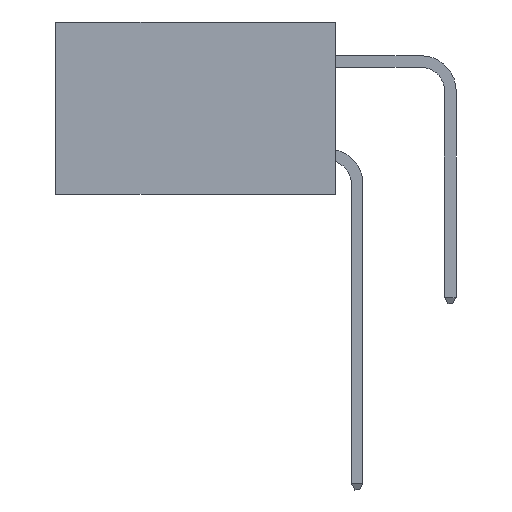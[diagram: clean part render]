
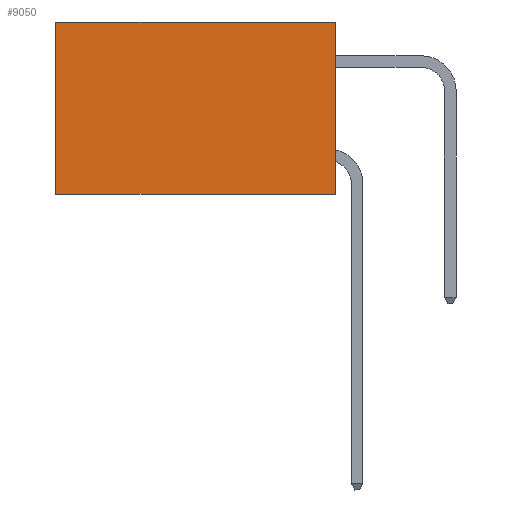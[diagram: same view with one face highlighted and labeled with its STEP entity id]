
A CAD part, left-side view. The second image highlights one B-rep face of the part: STEP entity #9050.
In plain terms, the highlighted planar face has unit normal (-1, 0, 0).
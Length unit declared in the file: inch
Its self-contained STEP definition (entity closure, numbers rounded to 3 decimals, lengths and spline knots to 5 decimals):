
#246 = DIRECTION ( 'NONE',  ( 1., 0., 0. ) ) ;
#2135 = CARTESIAN_POINT ( 'NONE',  ( 0.2875, 0.6, -0.37 ) ) ;
#3579 = VERTEX_POINT ( 'NONE', #6731 ) ;
#5837 = ORIENTED_EDGE ( 'NONE', *, *, #15060, .T. ) ;
#6731 = CARTESIAN_POINT ( 'NONE',  ( 0.2875, 0., -0.37 ) ) ;
#9050 = ADVANCED_FACE ( 'NONE', ( #21233 ), #11220, .F. ) ;
#9184 = DIRECTION ( 'NONE',  ( 0., 1., 0. ) ) ;
#10200 = CARTESIAN_POINT ( 'NONE',  ( 0.2875, 0., 0. ) ) ;
#10990 = DIRECTION ( 'NONE',  ( 0., 0., -1. ) ) ;
#11158 = DIRECTION ( 'NONE',  ( 0., 0., -1. ) ) ;
#11220 = PLANE ( 'NONE',  #15817 ) ;
#11333 = EDGE_CURVE ( 'NONE', #24802, #27019, #31255, .T. ) ;
#13932 = CARTESIAN_POINT ( 'NONE',  ( 0.2875, 0., 0. ) ) ;
#15060 = EDGE_CURVE ( 'NONE', #20950, #24802, #25091, .T. ) ;
#15817 = AXIS2_PLACEMENT_3D ( 'NONE', #13932, #246, #10990 ) ;
#18059 = VECTOR ( 'NONE', #9184, 39.37008 ) ;
#20950 = VERTEX_POINT ( 'NONE', #10200 ) ;
#21134 = LINE ( 'NONE', #26355, #30874 ) ;
#21140 = ORIENTED_EDGE ( 'NONE', *, *, #22126, .F. ) ;
#21233 = FACE_OUTER_BOUND ( 'NONE', #25511, .T. ) ;
#22126 = EDGE_CURVE ( 'NONE', #3579, #27019, #22269, .T. ) ;
#22269 = LINE ( 'NONE', #30730, #18059 ) ;
#22641 = ORIENTED_EDGE ( 'NONE', *, *, #28471, .F. ) ;
#24246 = VECTOR ( 'NONE', #27109, 39.37008 ) ;
#24802 = VERTEX_POINT ( 'NONE', #33376 ) ;
#25091 = LINE ( 'NONE', #26993, #24246 ) ;
#25511 = EDGE_LOOP ( 'NONE', ( #26576, #21140, #22641, #5837 ) ) ;
#26355 = CARTESIAN_POINT ( 'NONE',  ( 0.2875, 0., 0. ) ) ;
#26576 = ORIENTED_EDGE ( 'NONE', *, *, #11333, .T. ) ;
#26993 = CARTESIAN_POINT ( 'NONE',  ( 0.2875, 0., 0. ) ) ;
#27019 = VERTEX_POINT ( 'NONE', #2135 ) ;
#27109 = DIRECTION ( 'NONE',  ( 0., 1., 0. ) ) ;
#28471 = EDGE_CURVE ( 'NONE', #20950, #3579, #21134, .T. ) ;
#28946 = DIRECTION ( 'NONE',  ( 0., 0., -1. ) ) ;
#30730 = CARTESIAN_POINT ( 'NONE',  ( 0.2875, 0., -0.37 ) ) ;
#30874 = VECTOR ( 'NONE', #28946, 39.37008 ) ;
#31255 = LINE ( 'NONE', #32989, #33819 ) ;
#32989 = CARTESIAN_POINT ( 'NONE',  ( 0.2875, 0.6, 0. ) ) ;
#33376 = CARTESIAN_POINT ( 'NONE',  ( 0.2875, 0.6, 0. ) ) ;
#33819 = VECTOR ( 'NONE', #11158, 39.37008 ) ;
